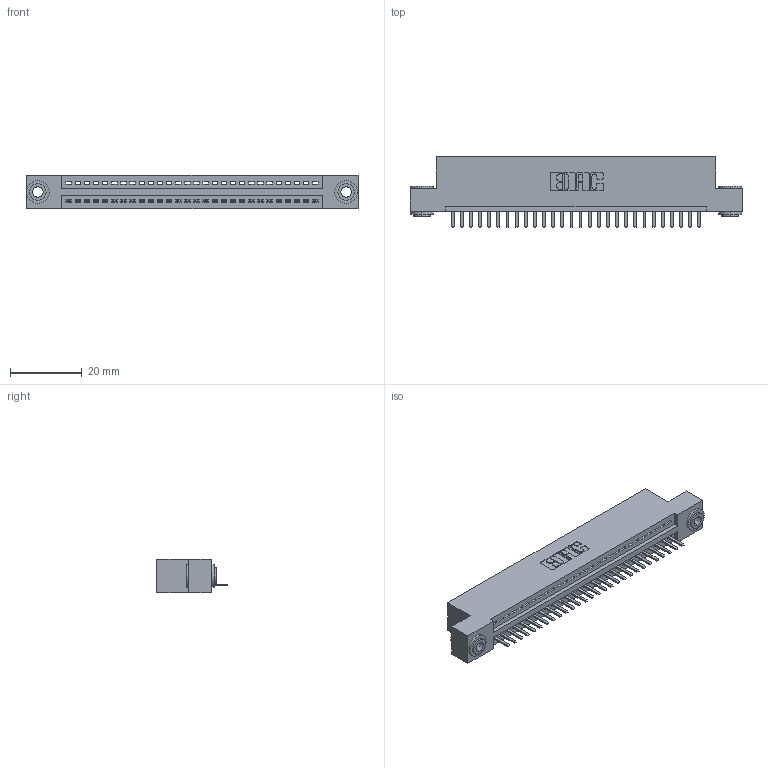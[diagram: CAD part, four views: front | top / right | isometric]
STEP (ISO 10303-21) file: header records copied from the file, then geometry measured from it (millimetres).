
FILE_DESCRIPTION (( 'STEP AP203' ), '1' );
FILE_NAME ('345-028-520-103.STEP', '2019-10-07T04:56:40', ( '' ), ( '' ), 'SwSTEP 2.0', 'SolidWorks 2016', '' );
FILE_SCHEMA (( 'CONFIG_CONTROL_DESIGN' ));
Length unit declared in the file: inch
Products named in the file (4): 345-292-001_345-293-120; 345 Part_Flush Mounting Lugs - 0.156 Dia-TH; 345-028-520-103; 345-250-002_345-250-002-102
Assembly tree (31 placements, depth 2):
  345-028-520-103
    345 Part_Flush Mounting Lugs - 0.156 Dia-TH
    345-292-001_345-293-120  x28
    345-250-002_345-250-002-102  x2
Bounding box: 92.33 x 19.68 x 9.4 mm (x, y, z)
Volume: 8593.7 mm3; surface area: 11180.9 mm2
Topology: 31 solids, 31 shells, 1900 faces, 5569 edges, 3634 vertices
Faces by surface type: plane 1266, cylinder 626, cone 8
Entity records: 23722 total; most frequent: CARTESIAN_POINT 4099, ORIENTED_EDGE 4042, DIRECTION 3619, EDGE_CURVE 2021, LINE 1749, VECTOR 1749, VERTEX_POINT 1342, AXIS2_PLACEMENT_3D 935
